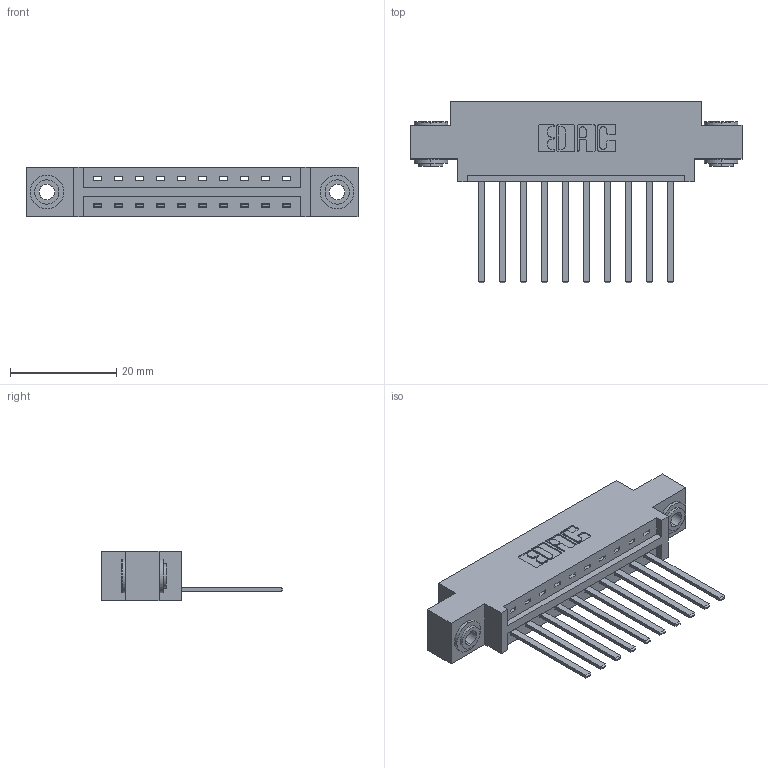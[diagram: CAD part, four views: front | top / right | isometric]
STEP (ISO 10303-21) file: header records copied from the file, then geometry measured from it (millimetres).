
FILE_DESCRIPTION (( 'STEP AP203' ), '1' );
FILE_NAME ('387-010-544-603.STEP', '2019-10-02T11:41:17', ( '' ), ( '' ), 'SwSTEP 2.0', 'SolidWorks 2016', '' );
FILE_SCHEMA (( 'CONFIG_CONTROL_DESIGN' ));
Length unit declared in the file: inch
Products named in the file (4): 387-010-544-603; 345-250-002_345-250-002-102; 345-292-001_345-293-144; 337 Part_0.170 Offset - 0.156 Dia-TH
Assembly tree (13 placements, depth 2):
  387-010-544-603
    337 Part_0.170 Offset - 0.156 Dia-TH
    345-292-001_345-293-144  x10
    345-250-002_345-250-002-102  x2
Bounding box: 62.64 x 34.3 x 9.4 mm (x, y, z)
Volume: 6127.3 mm3; surface area: 6864.1 mm2
Topology: 13 solids, 13 shells, 716 faces, 2099 edges, 1382 vertices
Faces by surface type: plane 504, cylinder 204, cone 8
Entity records: 12170 total; most frequent: CARTESIAN_POINT 2095, ORIENTED_EDGE 2034, DIRECTION 1859, EDGE_CURVE 1017, VECTOR 869, LINE 869, VERTEX_POINT 674, AXIS2_PLACEMENT_3D 495
